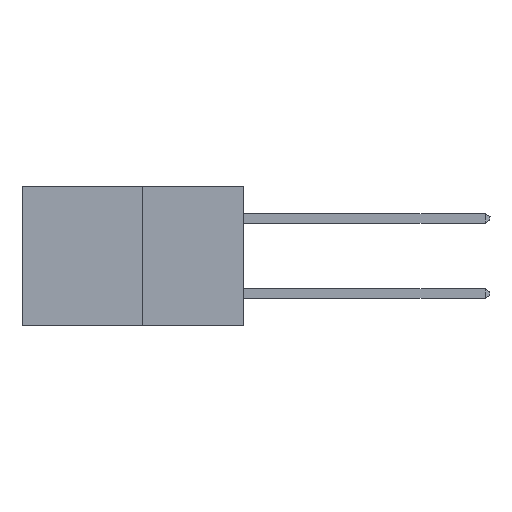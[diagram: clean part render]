
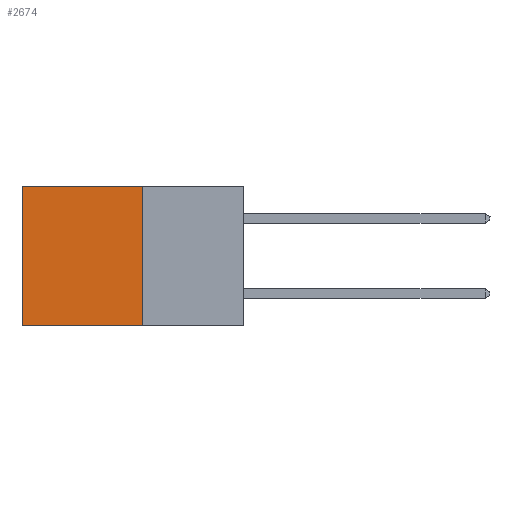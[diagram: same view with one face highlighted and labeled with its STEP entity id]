
A CAD part, left-side view. The second image highlights one B-rep face of the part: STEP entity #2674.
In plain terms, the highlighted planar face has unit normal (-1, 0, 0).
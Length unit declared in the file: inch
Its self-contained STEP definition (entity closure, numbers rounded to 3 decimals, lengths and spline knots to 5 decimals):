
#353 = VECTOR ( 'NONE', #2152, 39.37008 ) ;
#882 = ORIENTED_EDGE ( 'NONE', *, *, #6479, .T. ) ;
#1992 = VERTEX_POINT ( 'NONE', #4949 ) ;
#2152 = DIRECTION ( 'NONE',  ( 0., 0., -1. ) ) ;
#2295 = DIRECTION ( 'NONE',  ( 0., 0., -1. ) ) ;
#2321 = DIRECTION ( 'NONE',  ( 1., 0., 0. ) ) ;
#2347 = PLANE ( 'NONE',  #9049 ) ;
#2465 = CARTESIAN_POINT ( 'NONE',  ( 0.277, 0.27, -0.37 ) ) ;
#2674 = ADVANCED_FACE ( 'NONE', ( #8920 ), #2347, .F. ) ;
#3537 = VECTOR ( 'NONE', #4690, 39.37008 ) ;
#3814 = LINE ( 'NONE', #19752, #19634 ) ;
#4140 = CARTESIAN_POINT ( 'NONE',  ( 0.277, 0.27, -0.37 ) ) ;
#4437 = CARTESIAN_POINT ( 'NONE',  ( 0.277, 0.59, -0.37 ) ) ;
#4489 = ORIENTED_EDGE ( 'NONE', *, *, #12125, .T. ) ;
#4531 = DIRECTION ( 'NONE',  ( 0., 1., 0. ) ) ;
#4690 = DIRECTION ( 'NONE',  ( 0., 0., -1. ) ) ;
#4949 = CARTESIAN_POINT ( 'NONE',  ( 0.277, 0.27, 0. ) ) ;
#6411 = ORIENTED_EDGE ( 'NONE', *, *, #13091, .F. ) ;
#6479 = EDGE_CURVE ( 'NONE', #1992, #16556, #3814, .T. ) ;
#7013 = VECTOR ( 'NONE', #4531, 39.37008 ) ;
#7073 = VERTEX_POINT ( 'NONE', #17485 ) ;
#7116 = EDGE_CURVE ( 'NONE', #1992, #7073, #12737, .T. ) ;
#7511 = LINE ( 'NONE', #4140, #7013 ) ;
#7753 = LINE ( 'NONE', #4437, #3537 ) ;
#8920 = FACE_OUTER_BOUND ( 'NONE', #17202, .T. ) ;
#8990 = ORIENTED_EDGE ( 'NONE', *, *, #7116, .F. ) ;
#9049 = AXIS2_PLACEMENT_3D ( 'NONE', #2465, #2321, #2295 ) ;
#12125 = EDGE_CURVE ( 'NONE', #16556, #13794, #7753, .T. ) ;
#12737 = LINE ( 'NONE', #17813, #353 ) ;
#12791 = CARTESIAN_POINT ( 'NONE',  ( 0.277, 0.59, -0.37 ) ) ;
#13091 = EDGE_CURVE ( 'NONE', #7073, #13794, #7511, .T. ) ;
#13794 = VERTEX_POINT ( 'NONE', #12791 ) ;
#16556 = VERTEX_POINT ( 'NONE', #19054 ) ;
#17202 = EDGE_LOOP ( 'NONE', ( #4489, #6411, #8990, #882 ) ) ;
#17485 = CARTESIAN_POINT ( 'NONE',  ( 0.277, 0.27, -0.37 ) ) ;
#17813 = CARTESIAN_POINT ( 'NONE',  ( 0.277, 0.27, -0.37 ) ) ;
#18952 = DIRECTION ( 'NONE',  ( 0., 1., 0. ) ) ;
#19054 = CARTESIAN_POINT ( 'NONE',  ( 0.277, 0.59, 0. ) ) ;
#19634 = VECTOR ( 'NONE', #18952, 39.37008 ) ;
#19752 = CARTESIAN_POINT ( 'NONE',  ( 0.277, 0.27, 0. ) ) ;
